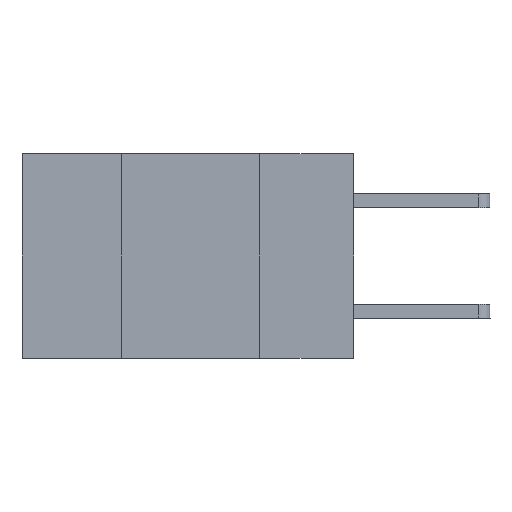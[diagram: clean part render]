
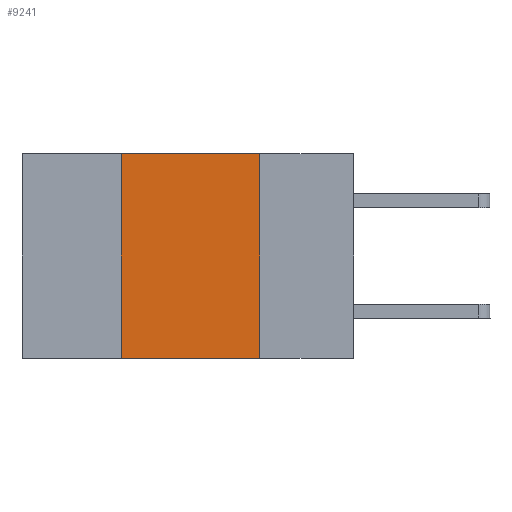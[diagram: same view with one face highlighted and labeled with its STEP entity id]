
A CAD part, left-side view. The second image highlights one B-rep face of the part: STEP entity #9241.
In plain terms, the highlighted planar face has unit normal (-1, 0, 0).
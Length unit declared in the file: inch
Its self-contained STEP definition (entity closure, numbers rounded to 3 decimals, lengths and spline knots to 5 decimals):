
#294 = EDGE_CURVE ( 'NONE', #961, #4874, #2036, .T. ) ;
#683 = VECTOR ( 'NONE', #4530, 39.37008 ) ;
#961 = VERTEX_POINT ( 'NONE', #9726 ) ;
#969 = DIRECTION ( 'NONE',  ( 0., 0., -1. ) ) ;
#1245 = EDGE_CURVE ( 'NONE', #961, #4414, #8508, .T. ) ;
#1261 = DIRECTION ( 'NONE',  ( 0., -1., 0. ) ) ;
#1290 = CARTESIAN_POINT ( 'NONE',  ( 0., 0.6, 0. ) ) ;
#1338 = ORIENTED_EDGE ( 'NONE', *, *, #1245, .T. ) ;
#1579 = CARTESIAN_POINT ( 'NONE',  ( 0., 0.42, 0. ) ) ;
#2036 = LINE ( 'NONE', #2417, #2157 ) ;
#2157 = VECTOR ( 'NONE', #8687, 39.37008 ) ;
#2201 = CARTESIAN_POINT ( 'NONE',  ( 0., 0.17, 0. ) ) ;
#2357 = VECTOR ( 'NONE', #1261, 39.37008 ) ;
#2417 = CARTESIAN_POINT ( 'NONE',  ( 0., 0.42, 0. ) ) ;
#2820 = DIRECTION ( 'NONE',  ( 1., 0., 0. ) ) ;
#2960 = CARTESIAN_POINT ( 'NONE',  ( 0., 0.17, -0.37 ) ) ;
#3510 = EDGE_LOOP ( 'NONE', ( #3898, #9457, #7250, #1338 ) ) ;
#3699 = EDGE_CURVE ( 'NONE', #7418, #4414, #9229, .T. ) ;
#3712 = PLANE ( 'NONE',  #8440 ) ;
#3898 = ORIENTED_EDGE ( 'NONE', *, *, #3699, .F. ) ;
#4414 = VERTEX_POINT ( 'NONE', #2960 ) ;
#4530 = DIRECTION ( 'NONE',  ( 0., -1., 0. ) ) ;
#4874 = VERTEX_POINT ( 'NONE', #1579 ) ;
#4957 = CARTESIAN_POINT ( 'NONE',  ( 0., 0.6, 0. ) ) ;
#6013 = VECTOR ( 'NONE', #969, 39.37008 ) ;
#7250 = ORIENTED_EDGE ( 'NONE', *, *, #294, .F. ) ;
#7418 = VERTEX_POINT ( 'NONE', #2201 ) ;
#8196 = EDGE_CURVE ( 'NONE', #4874, #7418, #8854, .T. ) ;
#8406 = DIRECTION ( 'NONE',  ( 0., 0., -1. ) ) ;
#8440 = AXIS2_PLACEMENT_3D ( 'NONE', #1290, #2820, #8406 ) ;
#8508 = LINE ( 'NONE', #9135, #683 ) ;
#8687 = DIRECTION ( 'NONE',  ( 0., 0., 1. ) ) ;
#8854 = LINE ( 'NONE', #4957, #2357 ) ;
#9135 = CARTESIAN_POINT ( 'NONE',  ( 0., 0.6, -0.37 ) ) ;
#9229 = LINE ( 'NONE', #9508, #6013 ) ;
#9241 = ADVANCED_FACE ( 'NONE', ( #9458 ), #3712, .F. ) ;
#9457 = ORIENTED_EDGE ( 'NONE', *, *, #8196, .F. ) ;
#9458 = FACE_OUTER_BOUND ( 'NONE', #3510, .T. ) ;
#9508 = CARTESIAN_POINT ( 'NONE',  ( 0., 0.17, 0. ) ) ;
#9726 = CARTESIAN_POINT ( 'NONE',  ( 0., 0.42, -0.37 ) ) ;
